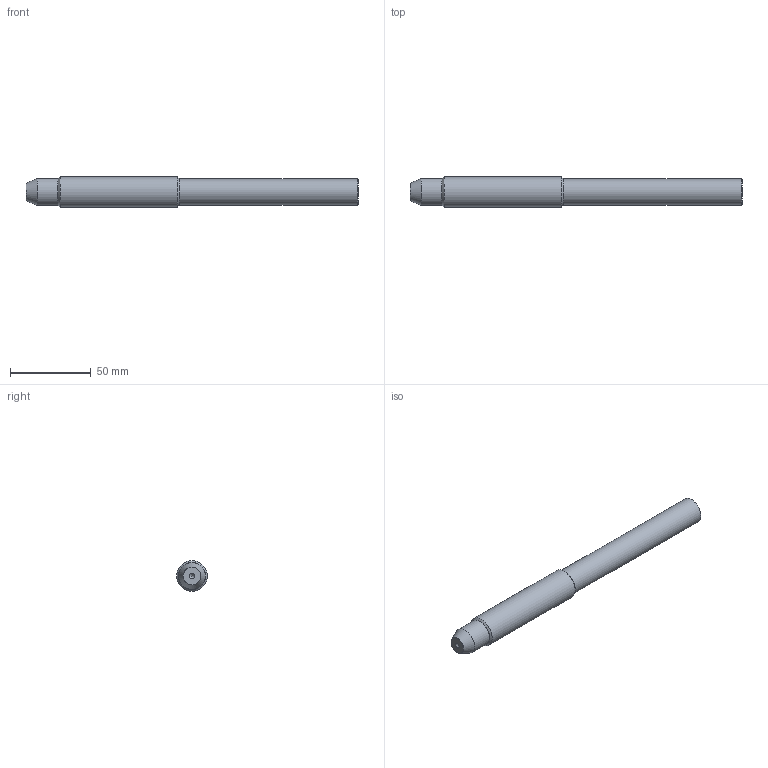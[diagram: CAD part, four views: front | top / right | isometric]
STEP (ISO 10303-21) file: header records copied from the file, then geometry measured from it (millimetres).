
FILE_DESCRIPTION(/* description */ (''),/* implementation_level */ '2;1');
FILE_NAME(/* author */ (''),/* organization */ (''),/* preprocessor_version */ 'ST-DEVELOPER v15.2',/* originating_system */ 'Autodesk Translator Framework v2.0.0.5431',/* authorisation */ '');
FILE_SCHEMA (('AUTOMOTIVE_DESIGN { 1 0 10303 214 3 1 1 }'));
Length unit declared in the file: centimetre
Products named in the file (1): (Unsaved)
Bounding box: 206 x 19 x 19 mm (x, y, z)
Volume: 48254.9 mm3; surface area: 11518.5 mm2
Topology: 1 solids, 1 shells, 14 faces, 33 edges, 21 vertices
Faces by surface type: cone 6, cylinder 3, torus 2, plane 2, bspline 1
Full cylindrical faces by diameter (mm): 16.3 x1, 16.7 x1, 19 x1
Entity records: 352 total; most frequent: CARTESIAN_POINT 97, DIRECTION 53, ORIENTED_EDGE 30, AXIS2_PLACEMENT_3D 26, EDGE_LOOP 25, EDGE_CURVE 15, FACE_OUTER_BOUND 14, VERTEX_POINT 14
